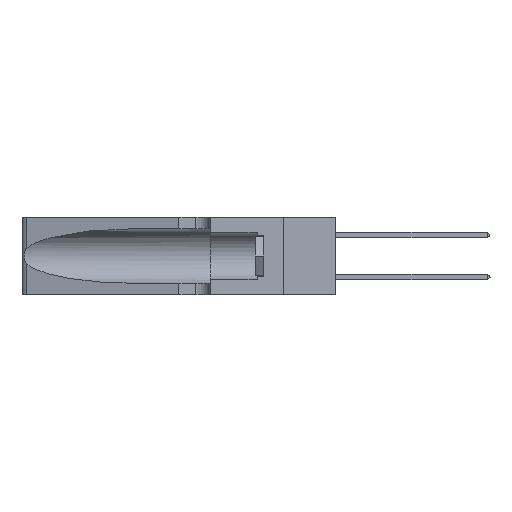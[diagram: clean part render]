
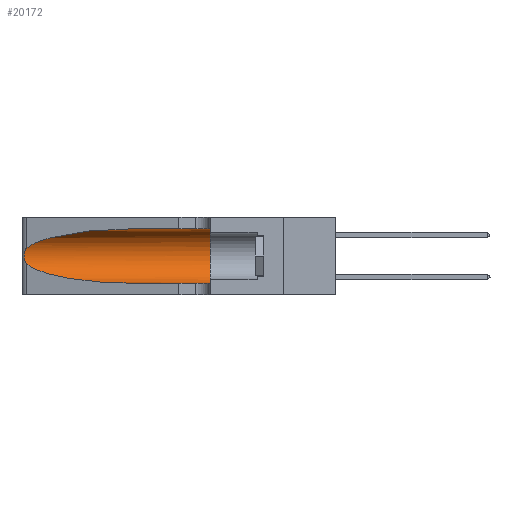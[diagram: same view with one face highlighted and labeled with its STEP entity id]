
A CAD part, left-side view. The second image highlights one B-rep face of the part: STEP entity #20172.
In plain terms, the highlighted cylindrical face has radius 3.308 mm (diameter 6.617 mm), a partial arc.
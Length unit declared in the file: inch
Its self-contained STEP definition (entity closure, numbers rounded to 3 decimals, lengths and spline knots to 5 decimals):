
#77 = DIRECTION ( 'NONE',  ( 0., 0., -1. ) ) ;
#335 = EDGE_CURVE ( 'NONE', #8807, #21578, #10353, .T. ) ;
#624 = CARTESIAN_POINT ( 'NONE',  ( 0.25789, 1.23486, 0.15765 ) ) ;
#1179 = FACE_OUTER_BOUND ( 'NONE', #1579, .T. ) ;
#1579 = EDGE_LOOP ( 'NONE', ( #4679, #23223, #2963, #8964, #20296, #15242 ) ) ;
#2329 = CYLINDRICAL_SURFACE ( 'NONE', #16440, 0.13025 ) ;
#2388 = CARTESIAN_POINT ( 'NONE',  ( 0.25555, 1.22994, 0.2215 ) ) ;
#2554 = EDGE_CURVE ( 'NONE', #9325, #18798, #9082, .T. ) ;
#2711 = CARTESIAN_POINT ( 'NONE',  ( 0.25854, 1.2359, 0.20912 ) ) ;
#2963 = ORIENTED_EDGE ( 'NONE', *, *, #20494, .T. ) ;
#3048 = CARTESIAN_POINT ( 'NONE',  ( 0.2373, 1.15595, 0.08982 ) ) ;
#3427 = CARTESIAN_POINT ( 'NONE',  ( 0.1305, 1.61858, 0.185 ) ) ;
#3439 = DIRECTION ( 'NONE',  ( 0., -1., 0. ) ) ;
#3768 = AXIS2_PLACEMENT_3D ( 'NONE', #20583, #4092, #11529 ) ;
#4092 = DIRECTION ( 'NONE',  ( 0., 1., 0. ) ) ;
#4679 = ORIENTED_EDGE ( 'NONE', *, *, #6316, .T. ) ;
#5445 = DIRECTION ( 'NONE',  ( 0., -1., 0. ) ) ;
#6022 = CARTESIAN_POINT ( 'NONE',  ( 0.25856, 1.23593, 0.16098 ) ) ;
#6316 = EDGE_CURVE ( 'NONE', #8807, #22481, #6725, .T. ) ;
#6656 = CARTESIAN_POINT ( 'NONE',  ( 0.25487, 1.22718, 0.14631 ) ) ;
#6725 =( BOUNDED_CURVE ( )  B_SPLINE_CURVE ( 3, ( #22469, #14951, #16792, #7685 ),
 .UNSPECIFIED., .F., .T. ) 
 B_SPLINE_CURVE_WITH_KNOTS ( ( 4, 4 ),
 ( 1.5708, 2.84003 ),
 .UNSPECIFIED. ) 
 CURVE ( )  GEOMETRIC_REPRESENTATION_ITEM ( )  RATIONAL_B_SPLINE_CURVE ( ( 1., 0.87, 0.87, 1. ) ) 
 REPRESENTATION_ITEM ( '' )  );
#7261 = CARTESIAN_POINT ( 'NONE',  ( 0.1305, 0.35, 0.05475 ) ) ;
#7434 =( BOUNDED_CURVE ( )  B_SPLINE_CURVE ( 3, ( #6656, #3048, #19342, #20612 ),
 .UNSPECIFIED., .F., .T. ) 
 B_SPLINE_CURVE_WITH_KNOTS ( ( 4, 4 ),
 ( 3.44316, 4.71239 ),
 .UNSPECIFIED. ) 
 CURVE ( )  GEOMETRIC_REPRESENTATION_ITEM ( )  RATIONAL_B_SPLINE_CURVE ( ( 1., 0.87, 0.87, 1. ) ) 
 REPRESENTATION_ITEM ( '' )  );
#7685 = CARTESIAN_POINT ( 'NONE',  ( 0.25487, 1.22718, 0.22369 ) ) ;
#8698 = DIRECTION ( 'NONE',  ( 0., -1., 0. ) ) ;
#8807 = VERTEX_POINT ( 'NONE', #10060 ) ;
#8964 = ORIENTED_EDGE ( 'NONE', *, *, #2554, .T. ) ;
#9082 = LINE ( 'NONE', #15952, #22421 ) ;
#9325 = VERTEX_POINT ( 'NONE', #18142 ) ;
#9565 = CARTESIAN_POINT ( 'NONE',  ( 0.25787, 1.23484, 0.2124 ) ) ;
#9894 = CARTESIAN_POINT ( 'NONE',  ( 0.25555, 1.22993, 0.14849 ) ) ;
#10060 = CARTESIAN_POINT ( 'NONE',  ( 0.1305, 0.72297, 0.31525 ) ) ;
#10143 = CARTESIAN_POINT ( 'NONE',  ( 0.25487, 1.22718, 0.22369 ) ) ;
#10353 = LINE ( 'NONE', #21111, #15461 ) ;
#10892 = VERTEX_POINT ( 'NONE', #13618 ) ;
#11529 = DIRECTION ( 'NONE',  ( 0., 0., 1. ) ) ;
#13326 = CARTESIAN_POINT ( 'NONE',  ( 0.25487, 1.22718, 0.14631 ) ) ;
#13412 = B_SPLINE_CURVE_WITH_KNOTS ( 'NONE', 3,
 ( #22487, #2388, #20763, #9565, #2711, #22251, #22570, #17128, #18956, #6022, #624, #22410, #9894, #13326 ),
 .UNSPECIFIED., .F., .F.,
 ( 4, 2, 2, 2, 2, 2, 4 ),
 ( 0., 0.00027, 0.00053, 0.00107, 0.0016, 0.00187, 0.00214 ),
 .UNSPECIFIED. ) ;
#13618 = CARTESIAN_POINT ( 'NONE',  ( 0.25487, 1.22718, 0.14631 ) ) ;
#14656 = CIRCLE ( 'NONE', #3768, 0.13025 ) ;
#14951 = CARTESIAN_POINT ( 'NONE',  ( 0.18966, 0.96281, 0.31525 ) ) ;
#15242 = ORIENTED_EDGE ( 'NONE', *, *, #335, .F. ) ;
#15246 = CARTESIAN_POINT ( 'NONE',  ( 0.1305, 0.35, 0.31525 ) ) ;
#15461 = VECTOR ( 'NONE', #8698, 39.37008 ) ;
#15766 = EDGE_CURVE ( 'NONE', #21578, #18798, #14656, .T. ) ;
#15952 = CARTESIAN_POINT ( 'NONE',  ( 0.1305, 1.61858, 0.05475 ) ) ;
#16440 = AXIS2_PLACEMENT_3D ( 'NONE', #3427, #5445, #77 ) ;
#16792 = CARTESIAN_POINT ( 'NONE',  ( 0.2373, 1.15595, 0.28018 ) ) ;
#17020 = EDGE_CURVE ( 'NONE', #22481, #10892, #13412, .T. ) ;
#17128 = CARTESIAN_POINT ( 'NONE',  ( 0.26075, 1.23896, 0.178 ) ) ;
#18142 = CARTESIAN_POINT ( 'NONE',  ( 0.1305, 0.72297, 0.05475 ) ) ;
#18798 = VERTEX_POINT ( 'NONE', #7261 ) ;
#18956 = CARTESIAN_POINT ( 'NONE',  ( 0.26017, 1.23833, 0.17102 ) ) ;
#19342 = CARTESIAN_POINT ( 'NONE',  ( 0.18966, 0.96281, 0.05475 ) ) ;
#20172 = ADVANCED_FACE ( 'NONE', ( #1179 ), #2329, .F. ) ;
#20296 = ORIENTED_EDGE ( 'NONE', *, *, #15766, .F. ) ;
#20494 = EDGE_CURVE ( 'NONE', #10892, #9325, #7434, .T. ) ;
#20583 = CARTESIAN_POINT ( 'NONE',  ( 0.1305, 0.35, 0.185 ) ) ;
#20612 = CARTESIAN_POINT ( 'NONE',  ( 0.1305, 0.72297, 0.05475 ) ) ;
#20763 = CARTESIAN_POINT ( 'NONE',  ( 0.25639, 1.23184, 0.21858 ) ) ;
#21111 = CARTESIAN_POINT ( 'NONE',  ( 0.1305, 1.61858, 0.31525 ) ) ;
#21578 = VERTEX_POINT ( 'NONE', #15246 ) ;
#22251 = CARTESIAN_POINT ( 'NONE',  ( 0.26018, 1.23835, 0.19895 ) ) ;
#22410 = CARTESIAN_POINT ( 'NONE',  ( 0.25639, 1.23186, 0.15144 ) ) ;
#22421 = VECTOR ( 'NONE', #3439, 39.37008 ) ;
#22469 = CARTESIAN_POINT ( 'NONE',  ( 0.1305, 0.72297, 0.31525 ) ) ;
#22481 = VERTEX_POINT ( 'NONE', #10143 ) ;
#22487 = CARTESIAN_POINT ( 'NONE',  ( 0.25487, 1.22718, 0.22369 ) ) ;
#22570 = CARTESIAN_POINT ( 'NONE',  ( 0.26075, 1.23896, 0.19203 ) ) ;
#23223 = ORIENTED_EDGE ( 'NONE', *, *, #17020, .T. ) ;
